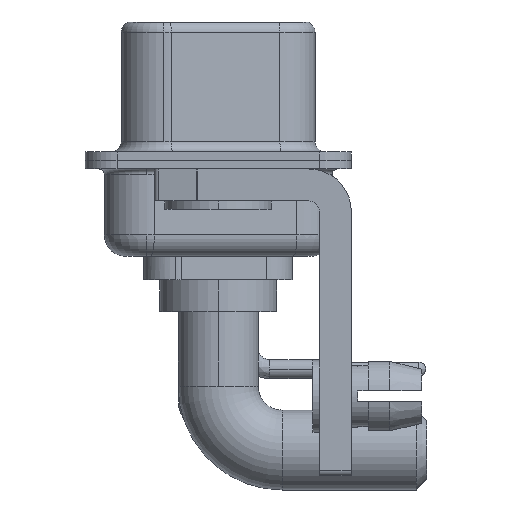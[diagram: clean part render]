
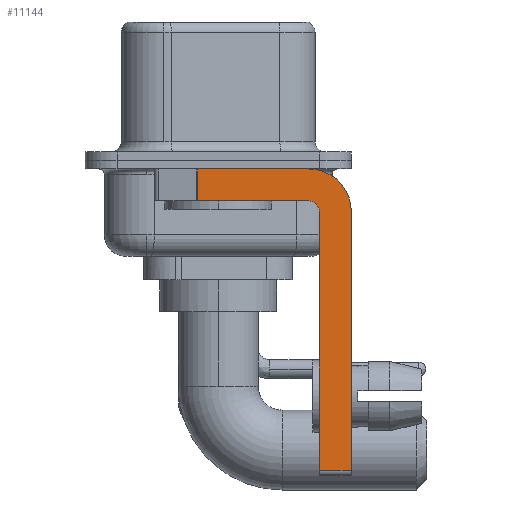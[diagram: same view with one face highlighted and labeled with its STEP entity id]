
A CAD part, left-side view. The second image highlights one B-rep face of the part: STEP entity #11144.
In plain terms, the highlighted planar face has unit normal (-1, 0, 0).
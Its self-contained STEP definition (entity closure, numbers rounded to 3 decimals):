
#183 = CARTESIAN_POINT ( 'NONE',  ( -2.9, -4.25, -0.4 ) ) ;
#1011 = FACE_OUTER_BOUND ( 'NONE', #14194, .T. ) ;
#1069 = LINE ( 'NONE', #1298, #3818 ) ;
#1216 = EDGE_CURVE ( 'NONE', #3693, #1848, #1654, .T. ) ;
#1298 = CARTESIAN_POINT ( 'NONE',  ( -2.9, -4.75, -14.8 ) ) ;
#1654 = LINE ( 'NONE', #11114, #16110 ) ;
#1750 = VERTEX_POINT ( 'NONE', #18730 ) ;
#1775 = DIRECTION ( 'NONE',  ( 0., 1., 0. ) ) ;
#1848 = VERTEX_POINT ( 'NONE', #16513 ) ;
#2057 = EDGE_CURVE ( 'NONE', #1750, #3693, #21387, .T. ) ;
#2771 = ORIENTED_EDGE ( 'NONE', *, *, #17557, .T. ) ;
#2803 = DIRECTION ( 'NONE',  ( 0., 0., -1. ) ) ;
#3083 = ORIENTED_EDGE ( 'NONE', *, *, #5031, .F. ) ;
#3137 = CARTESIAN_POINT ( 'NONE',  ( -2.9, -4.25, -2.4 ) ) ;
#3324 = CIRCLE ( 'NONE', #5629, 2. ) ;
#3462 = VERTEX_POINT ( 'NONE', #11475 ) ;
#3667 = CARTESIAN_POINT ( 'NONE',  ( -2.9, -6.25, -14.55 ) ) ;
#3693 = VERTEX_POINT ( 'NONE', #19359 ) ;
#3718 = CARTESIAN_POINT ( 'NONE',  ( -2.9, -4.75, -14.55 ) ) ;
#3818 = VECTOR ( 'NONE', #14070, 1000. ) ;
#5031 = EDGE_CURVE ( 'NONE', #19974, #15169, #22921, .T. ) ;
#5629 = AXIS2_PLACEMENT_3D ( 'NONE', #14978, #17097, #2803 ) ;
#5708 = ORIENTED_EDGE ( 'NONE', *, *, #19088, .F. ) ;
#6832 = CARTESIAN_POINT ( 'NONE',  ( -2.9, -4.25, -2.4 ) ) ;
#7034 = VECTOR ( 'NONE', #17173, 1000. ) ;
#7170 = DIRECTION ( 'NONE',  ( -1., 0., 0. ) ) ;
#7580 = LINE ( 'NONE', #20189, #13189 ) ;
#8013 = CARTESIAN_POINT ( 'NONE',  ( -2.9, -6.25, -2.4 ) ) ;
#8666 = VECTOR ( 'NONE', #15870, 1000. ) ;
#9796 = LINE ( 'NONE', #8013, #17302 ) ;
#9857 = VERTEX_POINT ( 'NONE', #3667 ) ;
#10352 = DIRECTION ( 'NONE',  ( 1., 0., 0. ) ) ;
#10711 = DIRECTION ( 'NONE',  ( 0., 0., 1. ) ) ;
#11114 = CARTESIAN_POINT ( 'NONE',  ( -2.9, -4.25, -1.9 ) ) ;
#11144 = ADVANCED_FACE ( 'NONE', ( #1011 ), #19295, .F. ) ;
#11475 = CARTESIAN_POINT ( 'NONE',  ( -2.9, -6.25, -2.4 ) ) ;
#11583 = DIRECTION ( 'NONE',  ( 0., -1., 0. ) ) ;
#12187 = ORIENTED_EDGE ( 'NONE', *, *, #1216, .F. ) ;
#12208 = LINE ( 'NONE', #21146, #7034 ) ;
#12669 = VERTEX_POINT ( 'NONE', #3718 ) ;
#12765 = ORIENTED_EDGE ( 'NONE', *, *, #16308, .F. ) ;
#12952 = EDGE_CURVE ( 'NONE', #19974, #1848, #12208, .T. ) ;
#13189 = VECTOR ( 'NONE', #11583, 1000. ) ;
#14070 = DIRECTION ( 'NONE',  ( 0., 0., 1. ) ) ;
#14194 = EDGE_LOOP ( 'NONE', ( #3083, #19327, #12187, #15539, #5708, #2771, #17850, #12765 ) ) ;
#14978 = CARTESIAN_POINT ( 'NONE',  ( -2.9, -4.25, -2.4 ) ) ;
#15169 = VERTEX_POINT ( 'NONE', #183 ) ;
#15266 = AXIS2_PLACEMENT_3D ( 'NONE', #3137, #10352, #21057 ) ;
#15539 = ORIENTED_EDGE ( 'NONE', *, *, #2057, .F. ) ;
#15870 = DIRECTION ( 'NONE',  ( 0., -1., 0. ) ) ;
#16110 = VECTOR ( 'NONE', #1775, 1000. ) ;
#16308 = EDGE_CURVE ( 'NONE', #15169, #3462, #3324, .T. ) ;
#16333 = EDGE_CURVE ( 'NONE', #3462, #9857, #9796, .T. ) ;
#16513 = CARTESIAN_POINT ( 'NONE',  ( -2.9, 0.978, -1.9 ) ) ;
#17097 = DIRECTION ( 'NONE',  ( 1., 0., 0. ) ) ;
#17173 = DIRECTION ( 'NONE',  ( 0., 0., -1. ) ) ;
#17219 = DIRECTION ( 'NONE',  ( 0., 0., -1. ) ) ;
#17302 = VECTOR ( 'NONE', #17219, 1000. ) ;
#17557 = EDGE_CURVE ( 'NONE', #12669, #9857, #7580, .T. ) ;
#17850 = ORIENTED_EDGE ( 'NONE', *, *, #16333, .F. ) ;
#18730 = CARTESIAN_POINT ( 'NONE',  ( -2.9, -4.75, -2.4 ) ) ;
#19088 = EDGE_CURVE ( 'NONE', #12669, #1750, #1069, .T. ) ;
#19295 = PLANE ( 'NONE',  #15266 ) ;
#19327 = ORIENTED_EDGE ( 'NONE', *, *, #12952, .T. ) ;
#19359 = CARTESIAN_POINT ( 'NONE',  ( -2.9, -4.25, -1.9 ) ) ;
#19393 = CARTESIAN_POINT ( 'NONE',  ( -2.9, 3., -0.4 ) ) ;
#19974 = VERTEX_POINT ( 'NONE', #20396 ) ;
#20189 = CARTESIAN_POINT ( 'NONE',  ( -2.9, -4.25, -14.55 ) ) ;
#20396 = CARTESIAN_POINT ( 'NONE',  ( -2.9, 0.978, -0.4 ) ) ;
#21057 = DIRECTION ( 'NONE',  ( 0., 0., -1. ) ) ;
#21146 = CARTESIAN_POINT ( 'NONE',  ( -2.9, 0.978, -1.9 ) ) ;
#21387 = CIRCLE ( 'NONE', #21763, 0.5 ) ;
#21763 = AXIS2_PLACEMENT_3D ( 'NONE', #6832, #7170, #10711 ) ;
#22921 = LINE ( 'NONE', #19393, #8666 ) ;
